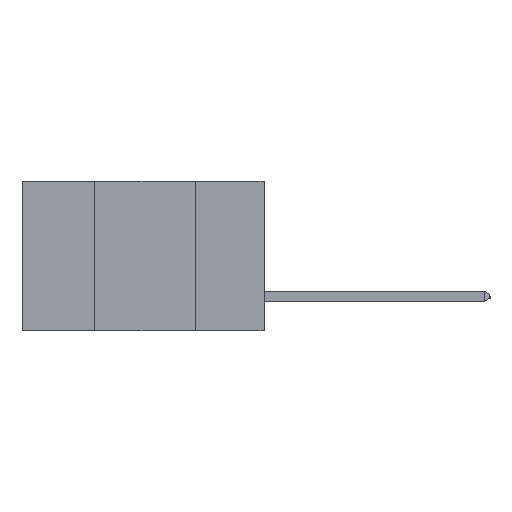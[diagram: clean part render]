
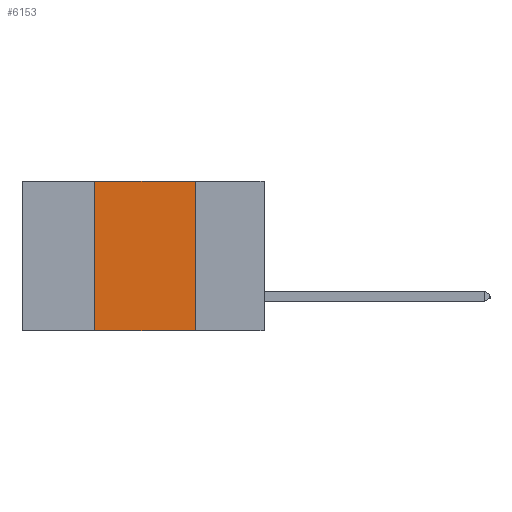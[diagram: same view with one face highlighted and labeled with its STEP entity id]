
A CAD part, left-side view. The second image highlights one B-rep face of the part: STEP entity #6153.
In plain terms, the highlighted planar face has unit normal (-1, 0, 0).
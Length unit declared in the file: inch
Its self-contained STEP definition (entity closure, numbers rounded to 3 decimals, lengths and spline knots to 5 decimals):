
#171 = CARTESIAN_POINT ( 'NONE',  ( 0., 0.17, -0.37 ) ) ;
#2513 = ORIENTED_EDGE ( 'NONE', *, *, #24054, .F. ) ;
#3423 = VERTEX_POINT ( 'NONE', #16328 ) ;
#3671 = LINE ( 'NONE', #13989, #26394 ) ;
#4656 = CARTESIAN_POINT ( 'NONE',  ( 0., 0.42, -0.37 ) ) ;
#6153 = ADVANCED_FACE ( 'NONE', ( #19349 ), #17956, .F. ) ;
#6680 = EDGE_LOOP ( 'NONE', ( #18179, #2513, #13945, #12900 ) ) ;
#9043 = DIRECTION ( 'NONE',  ( 0., 0., -1. ) ) ;
#9815 = EDGE_CURVE ( 'NONE', #28436, #19228, #13267, .T. ) ;
#10407 = LINE ( 'NONE', #19437, #28911 ) ;
#10416 = EDGE_CURVE ( 'NONE', #28436, #19130, #3671, .T. ) ;
#11914 = CARTESIAN_POINT ( 'NONE',  ( 0., 0.42, 0. ) ) ;
#12900 = ORIENTED_EDGE ( 'NONE', *, *, #9815, .T. ) ;
#13267 = LINE ( 'NONE', #23746, #25292 ) ;
#13299 = EDGE_CURVE ( 'NONE', #3423, #19228, #10407, .T. ) ;
#13945 = ORIENTED_EDGE ( 'NONE', *, *, #10416, .F. ) ;
#13989 = CARTESIAN_POINT ( 'NONE',  ( 0., 0.42, 0. ) ) ;
#14083 = DIRECTION ( 'NONE',  ( 0., 0., 1. ) ) ;
#14707 = DIRECTION ( 'NONE',  ( 0., 0., -1. ) ) ;
#15431 = VECTOR ( 'NONE', #22335, 39.37008 ) ;
#16328 = CARTESIAN_POINT ( 'NONE',  ( 0., 0.17, 0. ) ) ;
#17497 = CARTESIAN_POINT ( 'NONE',  ( 0., 0.6, 0. ) ) ;
#17956 = PLANE ( 'NONE',  #20627 ) ;
#18179 = ORIENTED_EDGE ( 'NONE', *, *, #13299, .F. ) ;
#19130 = VERTEX_POINT ( 'NONE', #11914 ) ;
#19228 = VERTEX_POINT ( 'NONE', #171 ) ;
#19349 = FACE_OUTER_BOUND ( 'NONE', #6680, .T. ) ;
#19437 = CARTESIAN_POINT ( 'NONE',  ( 0., 0.17, 0. ) ) ;
#20627 = AXIS2_PLACEMENT_3D ( 'NONE', #30508, #24240, #9043 ) ;
#22335 = DIRECTION ( 'NONE',  ( 0., -1., 0. ) ) ;
#22980 = DIRECTION ( 'NONE',  ( 0., -1., 0. ) ) ;
#23746 = CARTESIAN_POINT ( 'NONE',  ( 0., 0.6, -0.37 ) ) ;
#24054 = EDGE_CURVE ( 'NONE', #19130, #3423, #28275, .T. ) ;
#24240 = DIRECTION ( 'NONE',  ( 1., 0., 0. ) ) ;
#25292 = VECTOR ( 'NONE', #22980, 39.37008 ) ;
#26394 = VECTOR ( 'NONE', #14083, 39.37008 ) ;
#28275 = LINE ( 'NONE', #17497, #15431 ) ;
#28436 = VERTEX_POINT ( 'NONE', #4656 ) ;
#28911 = VECTOR ( 'NONE', #14707, 39.37008 ) ;
#30508 = CARTESIAN_POINT ( 'NONE',  ( 0., 0.6, 0. ) ) ;
